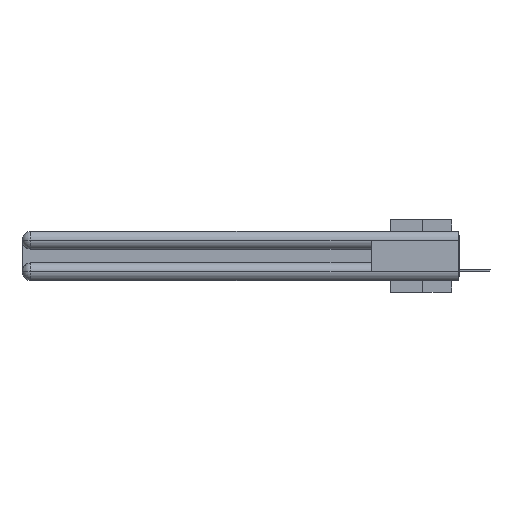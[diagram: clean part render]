
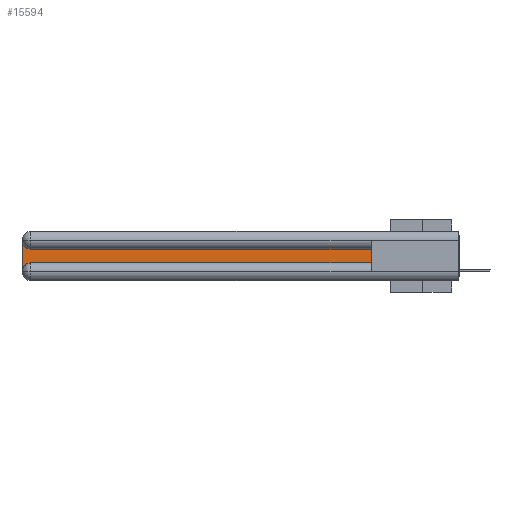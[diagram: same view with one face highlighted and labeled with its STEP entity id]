
A CAD part, left-side view. The second image highlights one B-rep face of the part: STEP entity #15594.
In plain terms, the highlighted planar face has unit normal (-1, 0, 0).
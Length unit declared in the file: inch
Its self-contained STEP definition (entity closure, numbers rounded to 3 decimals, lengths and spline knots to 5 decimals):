
#635 = CARTESIAN_POINT ( 'NONE',  ( 0.075, 3., -0.1225 ) ) ;
#2262 = VECTOR ( 'NONE', #7569, 39.37008 ) ;
#3619 = VECTOR ( 'NONE', #14400, 39.37008 ) ;
#3756 = VERTEX_POINT ( 'NONE', #20298 ) ;
#4178 = ORIENTED_EDGE ( 'NONE', *, *, #25683, .T. ) ;
#4692 = CIRCLE ( 'NONE', #11847, 0.06 ) ;
#5486 = CARTESIAN_POINT ( 'NONE',  ( 0.075, 2.94, -0.2175 ) ) ;
#5488 = CARTESIAN_POINT ( 'NONE',  ( 0.075, 0.6, -0.2175 ) ) ;
#6110 = CIRCLE ( 'NONE', #25040, 0.06 ) ;
#7569 = DIRECTION ( 'NONE',  ( 0., 1., 0. ) ) ;
#7750 = DIRECTION ( 'NONE',  ( 0., 0., 1. ) ) ;
#8668 = LINE ( 'NONE', #26226, #3619 ) ;
#8707 = CARTESIAN_POINT ( 'NONE',  ( 0.075, 2.94, -0.2775 ) ) ;
#9596 = PLANE ( 'NONE',  #20215 ) ;
#11847 = AXIS2_PLACEMENT_3D ( 'NONE', #35220, #14801, #17709 ) ;
#11909 = DIRECTION ( 'NONE',  ( 1., 0., 0. ) ) ;
#12560 = VERTEX_POINT ( 'NONE', #17535 ) ;
#12577 = ORIENTED_EDGE ( 'NONE', *, *, #32411, .T. ) ;
#14400 = DIRECTION ( 'NONE',  ( 0., -1., 0. ) ) ;
#14589 = DIRECTION ( 'NONE',  ( 0., 0., -1. ) ) ;
#14801 = DIRECTION ( 'NONE',  ( 1., 0., 0. ) ) ;
#14914 = DIRECTION ( 'NONE',  ( 0., 0., -1. ) ) ;
#15594 = ADVANCED_FACE ( 'NONE', ( #20278 ), #9596, .F. ) ;
#16333 = VECTOR ( 'NONE', #7750, 39.37008 ) ;
#16391 = VERTEX_POINT ( 'NONE', #22394 ) ;
#17535 = CARTESIAN_POINT ( 'NONE',  ( 0.075, 3., -0.0625 ) ) ;
#17655 = EDGE_CURVE ( 'NONE', #36830, #20574, #8668, .T. ) ;
#17709 = DIRECTION ( 'NONE',  ( 0., 0., -1. ) ) ;
#17733 = ORIENTED_EDGE ( 'NONE', *, *, #23103, .T. ) ;
#17822 = LINE ( 'NONE', #19561, #2262 ) ;
#19561 = CARTESIAN_POINT ( 'NONE',  ( 0.075, 0.6, -0.1225 ) ) ;
#20215 = AXIS2_PLACEMENT_3D ( 'NONE', #635, #26923, #29899 ) ;
#20278 = FACE_OUTER_BOUND ( 'NONE', #25125, .T. ) ;
#20298 = CARTESIAN_POINT ( 'NONE',  ( 0.075, 0.6, -0.1225 ) ) ;
#20574 = VERTEX_POINT ( 'NONE', #5488 ) ;
#21107 = VERTEX_POINT ( 'NONE', #31140 ) ;
#21711 = VECTOR ( 'NONE', #14914, 39.37008 ) ;
#21823 = ORIENTED_EDGE ( 'NONE', *, *, #17655, .T. ) ;
#22394 = CARTESIAN_POINT ( 'NONE',  ( 0.075, 2.94, -0.1225 ) ) ;
#22743 = ORIENTED_EDGE ( 'NONE', *, *, #37593, .T. ) ;
#23103 = EDGE_CURVE ( 'NONE', #16391, #12560, #4692, .T. ) ;
#25040 = AXIS2_PLACEMENT_3D ( 'NONE', #8707, #11909, #14589 ) ;
#25125 = EDGE_LOOP ( 'NONE', ( #12577, #17733, #22743, #4178, #21823, #33329 ) ) ;
#25683 = EDGE_CURVE ( 'NONE', #21107, #36830, #6110, .T. ) ;
#26226 = CARTESIAN_POINT ( 'NONE',  ( 0.075, 0.6, -0.2175 ) ) ;
#26923 = DIRECTION ( 'NONE',  ( 1., 0., 0. ) ) ;
#29899 = DIRECTION ( 'NONE',  ( 0., 0., -1. ) ) ;
#31140 = CARTESIAN_POINT ( 'NONE',  ( 0.075, 3., -0.2775 ) ) ;
#32006 = CARTESIAN_POINT ( 'NONE',  ( 0.075, 3., -0.2175 ) ) ;
#32411 = EDGE_CURVE ( 'NONE', #3756, #16391, #17822, .T. ) ;
#33164 = LINE ( 'NONE', #32006, #21711 ) ;
#33329 = ORIENTED_EDGE ( 'NONE', *, *, #36416, .T. ) ;
#34138 = LINE ( 'NONE', #36778, #16333 ) ;
#35220 = CARTESIAN_POINT ( 'NONE',  ( 0.075, 2.94, -0.0625 ) ) ;
#36416 = EDGE_CURVE ( 'NONE', #20574, #3756, #34138, .T. ) ;
#36778 = CARTESIAN_POINT ( 'NONE',  ( 0.075, 0.6, -0.2175 ) ) ;
#36830 = VERTEX_POINT ( 'NONE', #5486 ) ;
#37593 = EDGE_CURVE ( 'NONE', #12560, #21107, #33164, .T. ) ;
